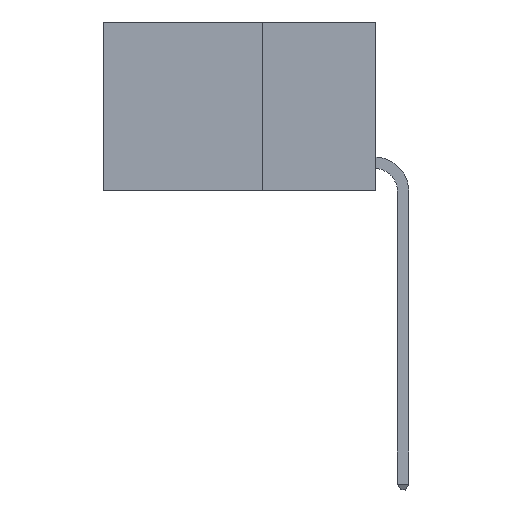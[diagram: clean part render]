
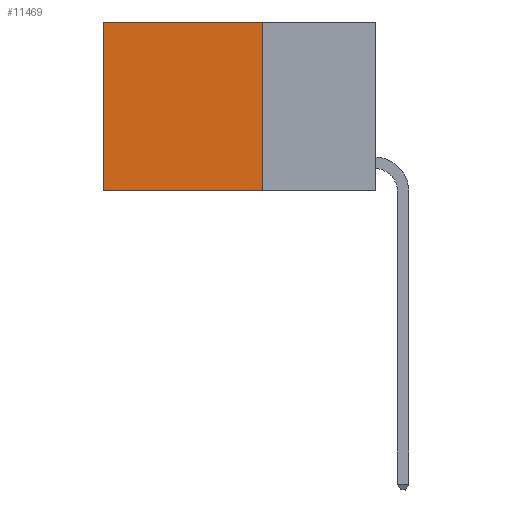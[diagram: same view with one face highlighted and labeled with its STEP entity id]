
A CAD part, left-side view. The second image highlights one B-rep face of the part: STEP entity #11469.
In plain terms, the highlighted planar face has unit normal (-1, 0, 0).
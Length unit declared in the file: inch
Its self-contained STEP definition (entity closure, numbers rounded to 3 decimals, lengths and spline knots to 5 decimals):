
#135 = LINE ( 'NONE', #13240, #11674 ) ;
#636 = EDGE_CURVE ( 'NONE', #18732, #25276, #135, .T. ) ;
#1558 = EDGE_CURVE ( 'NONE', #25276, #15562, #29462, .T. ) ;
#3491 = LINE ( 'NONE', #22932, #10350 ) ;
#3653 = VECTOR ( 'NONE', #14885, 39.37008 ) ;
#5480 = CARTESIAN_POINT ( 'NONE',  ( 0.2625, 0.25, 0. ) ) ;
#5494 = VECTOR ( 'NONE', #14316, 39.37008 ) ;
#8656 = CARTESIAN_POINT ( 'NONE',  ( 0.2625, 0.25, 0. ) ) ;
#9657 = CARTESIAN_POINT ( 'NONE',  ( 0.2625, 0.6, -0.37 ) ) ;
#10240 = CARTESIAN_POINT ( 'NONE',  ( 0.2625, 0.25, 0. ) ) ;
#10350 = VECTOR ( 'NONE', #25281, 39.37008 ) ;
#10972 = DIRECTION ( 'NONE',  ( 1., 0., 0. ) ) ;
#11469 = ADVANCED_FACE ( 'NONE', ( #24013 ), #22595, .F. ) ;
#11674 = VECTOR ( 'NONE', #17910, 39.37008 ) ;
#11968 = CARTESIAN_POINT ( 'NONE',  ( 0.2625, 0.6, 0. ) ) ;
#13240 = CARTESIAN_POINT ( 'NONE',  ( 0.2625, 0.25, 0. ) ) ;
#13681 = EDGE_LOOP ( 'NONE', ( #24131, #15775, #26123, #19476 ) ) ;
#14316 = DIRECTION ( 'NONE',  ( 0., 0., -1. ) ) ;
#14853 = CARTESIAN_POINT ( 'NONE',  ( 0.2625, 0.25, -0.37 ) ) ;
#14885 = DIRECTION ( 'NONE',  ( 0., 0., -1. ) ) ;
#15562 = VERTEX_POINT ( 'NONE', #9657 ) ;
#15733 = EDGE_CURVE ( 'NONE', #18732, #22804, #21452, .T. ) ;
#15775 = ORIENTED_EDGE ( 'NONE', *, *, #19019, .F. ) ;
#17061 = CARTESIAN_POINT ( 'NONE',  ( 0.2625, 0.6, 0. ) ) ;
#17910 = DIRECTION ( 'NONE',  ( 0., 1., 0. ) ) ;
#18732 = VERTEX_POINT ( 'NONE', #5480 ) ;
#19019 = EDGE_CURVE ( 'NONE', #22804, #15562, #3491, .T. ) ;
#19476 = ORIENTED_EDGE ( 'NONE', *, *, #636, .T. ) ;
#21452 = LINE ( 'NONE', #10240, #3653 ) ;
#22595 = PLANE ( 'NONE',  #24958 ) ;
#22804 = VERTEX_POINT ( 'NONE', #14853 ) ;
#22932 = CARTESIAN_POINT ( 'NONE',  ( 0.2625, 0.25, -0.37 ) ) ;
#24013 = FACE_OUTER_BOUND ( 'NONE', #13681, .T. ) ;
#24131 = ORIENTED_EDGE ( 'NONE', *, *, #1558, .T. ) ;
#24958 = AXIS2_PLACEMENT_3D ( 'NONE', #8656, #10972, #27257 ) ;
#25276 = VERTEX_POINT ( 'NONE', #17061 ) ;
#25281 = DIRECTION ( 'NONE',  ( 0., 1., 0. ) ) ;
#26123 = ORIENTED_EDGE ( 'NONE', *, *, #15733, .F. ) ;
#27257 = DIRECTION ( 'NONE',  ( 0., 0., -1. ) ) ;
#29462 = LINE ( 'NONE', #11968, #5494 ) ;
